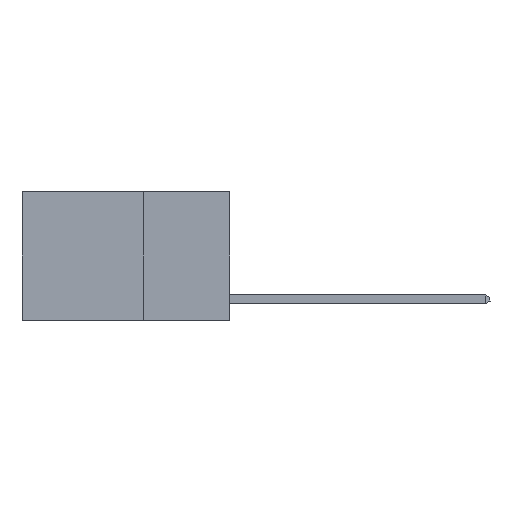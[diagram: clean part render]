
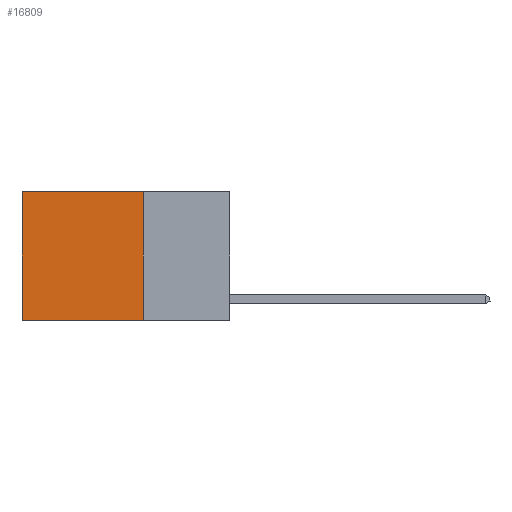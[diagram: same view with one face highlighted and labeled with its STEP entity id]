
A CAD part, left-side view. The second image highlights one B-rep face of the part: STEP entity #16809.
In plain terms, the highlighted planar face has unit normal (-1, 0, 0).
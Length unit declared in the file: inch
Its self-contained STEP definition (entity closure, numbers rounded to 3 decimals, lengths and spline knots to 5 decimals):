
#261 = VERTEX_POINT ( 'NONE', #19525 ) ;
#1476 = DIRECTION ( 'NONE',  ( 0., 1., 0. ) ) ;
#1740 = VECTOR ( 'NONE', #9241, 39.37008 ) ;
#1843 = CARTESIAN_POINT ( 'NONE',  ( 0.2625, 0.25, 0. ) ) ;
#1960 = ORIENTED_EDGE ( 'NONE', *, *, #9418, .T. ) ;
#2812 = EDGE_CURVE ( 'NONE', #261, #8785, #16276, .T. ) ;
#3115 = CARTESIAN_POINT ( 'NONE',  ( 0.2625, 0.25, 0. ) ) ;
#3767 = DIRECTION ( 'NONE',  ( 0., 1., 0. ) ) ;
#3833 = CARTESIAN_POINT ( 'NONE',  ( 0.2625, 0.25, 0. ) ) ;
#4778 = PLANE ( 'NONE',  #18794 ) ;
#6099 = ORIENTED_EDGE ( 'NONE', *, *, #2812, .T. ) ;
#6290 = DIRECTION ( 'NONE',  ( 0., 0., -1. ) ) ;
#6970 = LINE ( 'NONE', #7696, #1740 ) ;
#7696 = CARTESIAN_POINT ( 'NONE',  ( 0.2625, 0.25, 0. ) ) ;
#8785 = VERTEX_POINT ( 'NONE', #11146 ) ;
#9008 = LINE ( 'NONE', #12944, #19562 ) ;
#9241 = DIRECTION ( 'NONE',  ( 0., 0., -1. ) ) ;
#9277 = VECTOR ( 'NONE', #13431, 39.37008 ) ;
#9418 = EDGE_CURVE ( 'NONE', #17003, #261, #12934, .T. ) ;
#9610 = EDGE_LOOP ( 'NONE', ( #6099, #12945, #15216, #1960 ) ) ;
#10038 = VECTOR ( 'NONE', #1476, 39.37008 ) ;
#10297 = CARTESIAN_POINT ( 'NONE',  ( 0.2625, 0.6, 0. ) ) ;
#11146 = CARTESIAN_POINT ( 'NONE',  ( 0.2625, 0.6, -0.37 ) ) ;
#11483 = FACE_OUTER_BOUND ( 'NONE', #9610, .T. ) ;
#12490 = CARTESIAN_POINT ( 'NONE',  ( 0.2625, 0.25, -0.37 ) ) ;
#12934 = LINE ( 'NONE', #3115, #10038 ) ;
#12944 = CARTESIAN_POINT ( 'NONE',  ( 0.2625, 0.25, -0.37 ) ) ;
#12945 = ORIENTED_EDGE ( 'NONE', *, *, #19107, .F. ) ;
#13431 = DIRECTION ( 'NONE',  ( 0., 0., -1. ) ) ;
#14378 = EDGE_CURVE ( 'NONE', #17003, #16733, #6970, .T. ) ;
#15216 = ORIENTED_EDGE ( 'NONE', *, *, #14378, .F. ) ;
#15469 = DIRECTION ( 'NONE',  ( 1., 0., 0. ) ) ;
#16276 = LINE ( 'NONE', #10297, #9277 ) ;
#16733 = VERTEX_POINT ( 'NONE', #12490 ) ;
#16809 = ADVANCED_FACE ( 'NONE', ( #11483 ), #4778, .F. ) ;
#17003 = VERTEX_POINT ( 'NONE', #3833 ) ;
#18794 = AXIS2_PLACEMENT_3D ( 'NONE', #1843, #15469, #6290 ) ;
#19107 = EDGE_CURVE ( 'NONE', #16733, #8785, #9008, .T. ) ;
#19525 = CARTESIAN_POINT ( 'NONE',  ( 0.2625, 0.6, 0. ) ) ;
#19562 = VECTOR ( 'NONE', #3767, 39.37008 ) ;
